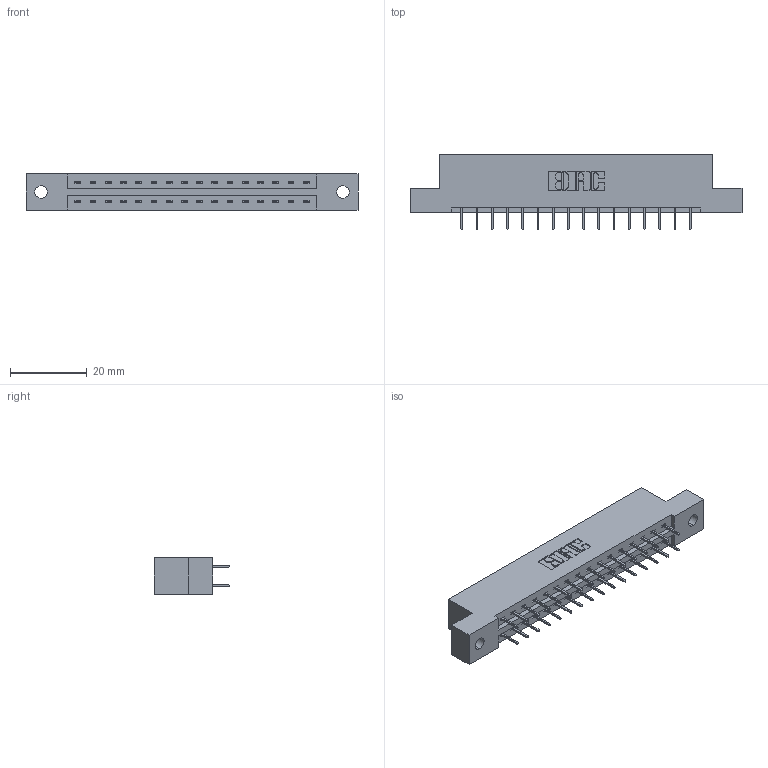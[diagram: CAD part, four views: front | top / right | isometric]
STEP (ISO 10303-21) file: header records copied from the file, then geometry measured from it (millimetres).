
FILE_DESCRIPTION (( 'STEP AP203' ), '1' );
FILE_NAME ('337-032-524-202.STEP', '2018-08-07T05:25:25', ( '' ), ( '' ), 'SwSTEP 2.0', 'SolidWorks 2016', '' );
FILE_SCHEMA (( 'CONFIG_CONTROL_DESIGN' ));
Length unit declared in the file: inch
Products named in the file (3): 337 Part_Flush Mounting Lugs - 0.128 Dia; 345-292-001_345-293-124; 337-032-524-202
Assembly tree (33 placements, depth 2):
  337-032-524-202
    337 Part_Flush Mounting Lugs - 0.128 Dia
    345-292-001_345-293-124  x32
Bounding box: 86.41 x 19.69 x 9.4 mm (x, y, z)
Volume: 8675.5 mm3; surface area: 9132.4 mm2
Topology: 33 solids, 33 shells, 1970 faces, 5591 edges, 3598 vertices
Faces by surface type: plane 1478, cylinder 492
Entity records: 15845 total; most frequent: CARTESIAN_POINT 2690, ORIENTED_EDGE 2626, DIRECTION 2337, EDGE_CURVE 1313, LINE 1189, VECTOR 1189, VERTEX_POINT 870, AXIS2_PLACEMENT_3D 574
